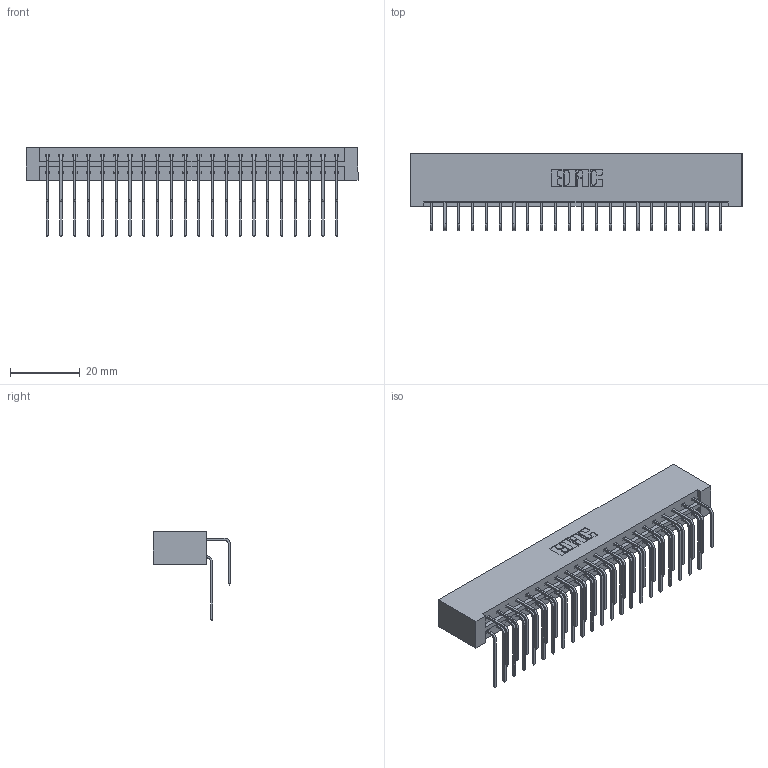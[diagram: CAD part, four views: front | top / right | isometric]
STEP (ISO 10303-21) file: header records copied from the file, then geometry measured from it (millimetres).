
FILE_DESCRIPTION (( 'STEP AP203' ), '1' );
FILE_NAME ('833-044-558-201.STEP', '2020-06-04T01:58:07', ( '' ), ( '' ), 'SwSTEP 2.0', 'SolidWorks 2020', '' );
FILE_SCHEMA (( 'CONFIG_CONTROL_DESIGN' ));
Length unit declared in the file: inch
Products named in the file (4): 833-044-558-201; 345-292-001_558 Tail - 2; 345-292-001_558 559 Tail - 1; 833 Part_Lugless
Assembly tree (45 placements, depth 2):
  833-044-558-201
    833 Part_Lugless
    345-292-001_558 559 Tail - 1  x22
    345-292-001_558 Tail - 2  x22
Bounding box: 95.43 x 22.17 x 25.53 mm (x, y, z)
Volume: 10441.6 mm3; surface area: 13418.4 mm2
Topology: 45 solids, 45 shells, 2482 faces, 7371 edges, 4854 vertices
Faces by surface type: plane 1738, cylinder 744
Entity records: 18247 total; most frequent: CARTESIAN_POINT 3097, ORIENTED_EDGE 2982, DIRECTION 2655, EDGE_CURVE 1491, LINE 1331, VECTOR 1331, VERTEX_POINT 990, AXIS2_PLACEMENT_3D 662
